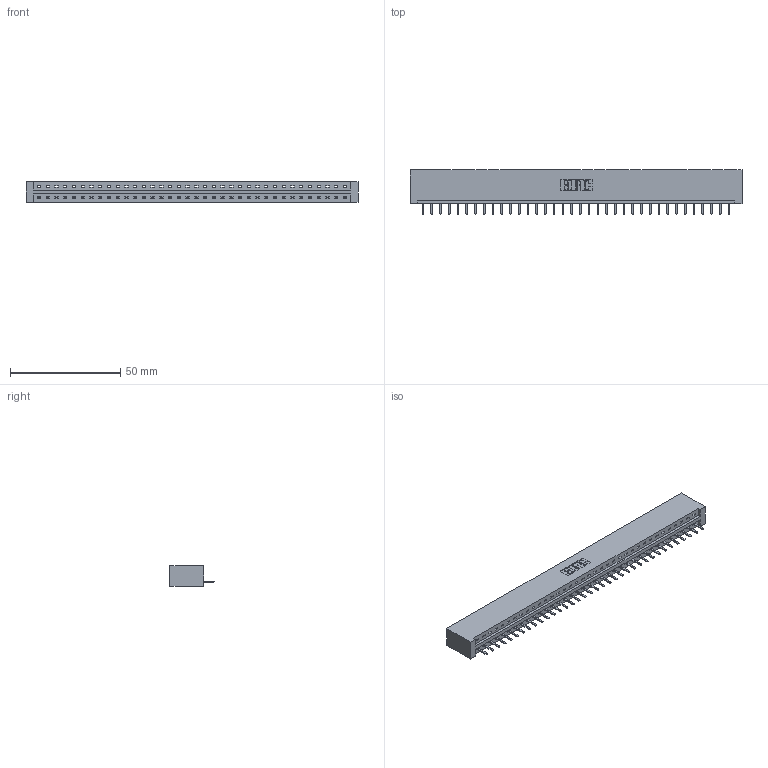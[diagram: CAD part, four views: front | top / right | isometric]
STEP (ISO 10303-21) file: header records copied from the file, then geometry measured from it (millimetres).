
FILE_DESCRIPTION (( 'STEP AP203' ), '1' );
FILE_NAME ('337-036-520-101.STEP', '2018-08-07T21:33:51', ( '' ), ( '' ), 'SwSTEP 2.0', 'SolidWorks 2016', '' );
FILE_SCHEMA (( 'CONFIG_CONTROL_DESIGN' ));
Length unit declared in the file: inch
Products named in the file (3): 337 Part_No Mounting Lugs; 345-292-001_345-293-120; 337-036-520-101
Assembly tree (37 placements, depth 2):
  337-036-520-101
    337 Part_No Mounting Lugs
    345-292-001_345-293-120  x36
Bounding box: 150.52 x 20.02 x 9.4 mm (x, y, z)
Volume: 16204.1 mm3; surface area: 16320 mm2
Topology: 37 solids, 37 shells, 2482 faces, 7343 edges, 4798 vertices
Faces by surface type: plane 1794, cylinder 688
Entity records: 27373 total; most frequent: CARTESIAN_POINT 4786, ORIENTED_EDGE 4746, DIRECTION 4021, EDGE_CURVE 2373, VECTOR 2249, LINE 2249, VERTEX_POINT 1578, AXIS2_PLACEMENT_3D 886
